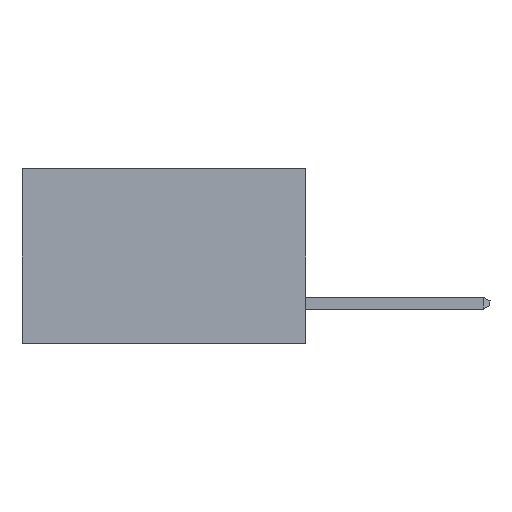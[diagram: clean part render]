
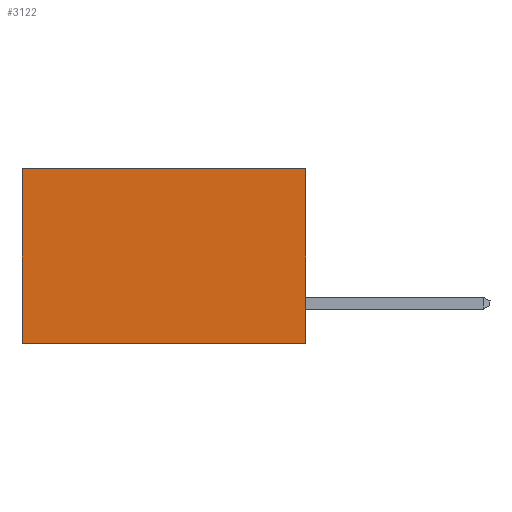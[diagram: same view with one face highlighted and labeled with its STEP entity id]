
A CAD part, left-side view. The second image highlights one B-rep face of the part: STEP entity #3122.
In plain terms, the highlighted planar face has unit normal (-1, 0, 0).
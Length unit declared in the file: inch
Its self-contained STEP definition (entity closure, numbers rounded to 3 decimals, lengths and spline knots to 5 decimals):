
#80 = DIRECTION ( 'NONE',  ( 0., 0., -1. ) ) ;
#232 = ORIENTED_EDGE ( 'NONE', *, *, #1001, .T. ) ;
#396 = DIRECTION ( 'NONE',  ( 0., 0., -1. ) ) ;
#548 = AXIS2_PLACEMENT_3D ( 'NONE', #4858, #975, #80 ) ;
#975 = DIRECTION ( 'NONE',  ( 1., 0., 0. ) ) ;
#1001 = EDGE_CURVE ( 'NONE', #2141, #3663, #3957, .T. ) ;
#1007 = CARTESIAN_POINT ( 'NONE',  ( 0.2615, 0., -0.37 ) ) ;
#1303 = CARTESIAN_POINT ( 'NONE',  ( 0.2615, 0.6, -0.37 ) ) ;
#1326 = DIRECTION ( 'NONE',  ( 0., 0., -1. ) ) ;
#1503 = EDGE_LOOP ( 'NONE', ( #8021, #6732, #2104, #232 ) ) ;
#1728 = FACE_OUTER_BOUND ( 'NONE', #1503, .T. ) ;
#1906 = VECTOR ( 'NONE', #396, 39.37008 ) ;
#2064 = CARTESIAN_POINT ( 'NONE',  ( 0.2615, 0.6, -0.37 ) ) ;
#2104 = ORIENTED_EDGE ( 'NONE', *, *, #7561, .F. ) ;
#2141 = VERTEX_POINT ( 'NONE', #3975 ) ;
#2196 = VECTOR ( 'NONE', #1326, 39.37008 ) ;
#3122 = ADVANCED_FACE ( 'NONE', ( #1728 ), #9397, .F. ) ;
#3501 = LINE ( 'NONE', #2064, #1906 ) ;
#3663 = VERTEX_POINT ( 'NONE', #9534 ) ;
#3957 = LINE ( 'NONE', #4701, #6297 ) ;
#3975 = CARTESIAN_POINT ( 'NONE',  ( 0.2615, 0., 0. ) ) ;
#4701 = CARTESIAN_POINT ( 'NONE',  ( 0.2615, 0., 0. ) ) ;
#4858 = CARTESIAN_POINT ( 'NONE',  ( 0.2615, 0., -0.37 ) ) ;
#5213 = CARTESIAN_POINT ( 'NONE',  ( 0.2615, 0., -0.37 ) ) ;
#5263 = DIRECTION ( 'NONE',  ( 0., 1., 0. ) ) ;
#6214 = LINE ( 'NONE', #9274, #8142 ) ;
#6297 = VECTOR ( 'NONE', #8551, 39.37008 ) ;
#6732 = ORIENTED_EDGE ( 'NONE', *, *, #7771, .F. ) ;
#7561 = EDGE_CURVE ( 'NONE', #2141, #9079, #8980, .T. ) ;
#7771 = EDGE_CURVE ( 'NONE', #9079, #9749, #6214, .T. ) ;
#8021 = ORIENTED_EDGE ( 'NONE', *, *, #9689, .T. ) ;
#8142 = VECTOR ( 'NONE', #5263, 39.37008 ) ;
#8551 = DIRECTION ( 'NONE',  ( 0., 1., 0. ) ) ;
#8980 = LINE ( 'NONE', #5213, #2196 ) ;
#9079 = VERTEX_POINT ( 'NONE', #1007 ) ;
#9274 = CARTESIAN_POINT ( 'NONE',  ( 0.2615, 0., -0.37 ) ) ;
#9397 = PLANE ( 'NONE',  #548 ) ;
#9534 = CARTESIAN_POINT ( 'NONE',  ( 0.2615, 0.6, 0. ) ) ;
#9689 = EDGE_CURVE ( 'NONE', #3663, #9749, #3501, .T. ) ;
#9749 = VERTEX_POINT ( 'NONE', #1303 ) ;
